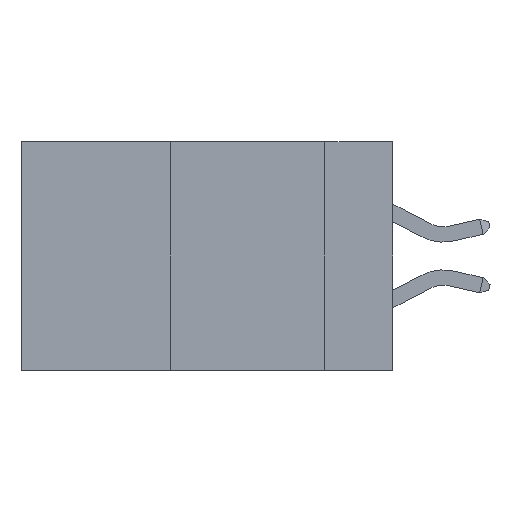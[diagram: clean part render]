
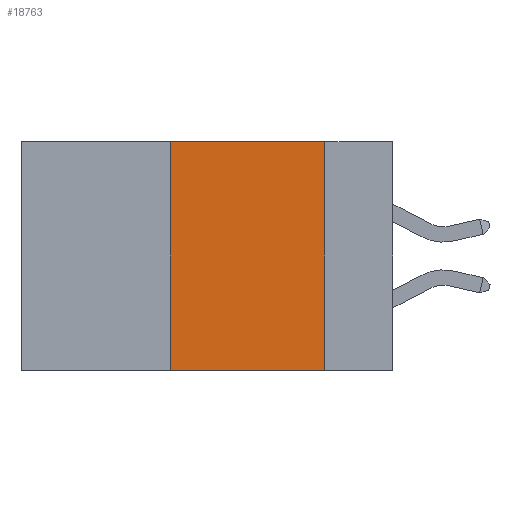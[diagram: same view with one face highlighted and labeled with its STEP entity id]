
A CAD part, left-side view. The second image highlights one B-rep face of the part: STEP entity #18763.
In plain terms, the highlighted planar face has unit normal (-1, 0, 0).
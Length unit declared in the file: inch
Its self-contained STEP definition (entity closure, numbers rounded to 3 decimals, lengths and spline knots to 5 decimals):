
#264 = VERTEX_POINT ( 'NONE', #22663 ) ;
#1376 = DIRECTION ( 'NONE',  ( 1., 0., 0. ) ) ;
#3195 = CARTESIAN_POINT ( 'NONE',  ( 0., 0.36, 0. ) ) ;
#3597 = CARTESIAN_POINT ( 'NONE',  ( 0., 0.6, -0.37 ) ) ;
#4513 = DIRECTION ( 'NONE',  ( 0., 0., -1. ) ) ;
#4616 = LINE ( 'NONE', #3597, #22181 ) ;
#5320 = VECTOR ( 'NONE', #4513, 39.37008 ) ;
#5803 = EDGE_CURVE ( 'NONE', #264, #16401, #4616, .T. ) ;
#6816 = AXIS2_PLACEMENT_3D ( 'NONE', #20392, #1376, #9915 ) ;
#7433 = CARTESIAN_POINT ( 'NONE',  ( 0., 0.11, 0. ) ) ;
#7488 = VECTOR ( 'NONE', #25372, 39.37008 ) ;
#7644 = VERTEX_POINT ( 'NONE', #3195 ) ;
#8243 = CARTESIAN_POINT ( 'NONE',  ( 0., 0.36, 0. ) ) ;
#8740 = VECTOR ( 'NONE', #18044, 39.37008 ) ;
#9915 = DIRECTION ( 'NONE',  ( 0., 0., -1. ) ) ;
#10943 = LINE ( 'NONE', #25445, #5320 ) ;
#11496 = VERTEX_POINT ( 'NONE', #7433 ) ;
#13374 = EDGE_LOOP ( 'NONE', ( #26297, #23035, #20560, #19013 ) ) ;
#13442 = CARTESIAN_POINT ( 'NONE',  ( 0., 0.11, -0.37 ) ) ;
#14347 = LINE ( 'NONE', #24248, #8740 ) ;
#15193 = EDGE_CURVE ( 'NONE', #11496, #16401, #10943, .T. ) ;
#16401 = VERTEX_POINT ( 'NONE', #13442 ) ;
#18044 = DIRECTION ( 'NONE',  ( 0., -1., 0. ) ) ;
#18763 = ADVANCED_FACE ( 'NONE', ( #23980 ), #22612, .F. ) ;
#19013 = ORIENTED_EDGE ( 'NONE', *, *, #5803, .T. ) ;
#19242 = EDGE_CURVE ( 'NONE', #7644, #11496, #14347, .T. ) ;
#20392 = CARTESIAN_POINT ( 'NONE',  ( 0., 0.6, 0. ) ) ;
#20560 = ORIENTED_EDGE ( 'NONE', *, *, #23405, .F. ) ;
#20727 = LINE ( 'NONE', #8243, #7488 ) ;
#22181 = VECTOR ( 'NONE', #23232, 39.37008 ) ;
#22612 = PLANE ( 'NONE',  #6816 ) ;
#22663 = CARTESIAN_POINT ( 'NONE',  ( 0., 0.36, -0.37 ) ) ;
#23035 = ORIENTED_EDGE ( 'NONE', *, *, #19242, .F. ) ;
#23232 = DIRECTION ( 'NONE',  ( 0., -1., 0. ) ) ;
#23405 = EDGE_CURVE ( 'NONE', #264, #7644, #20727, .T. ) ;
#23980 = FACE_OUTER_BOUND ( 'NONE', #13374, .T. ) ;
#24248 = CARTESIAN_POINT ( 'NONE',  ( 0., 0.6, 0. ) ) ;
#25372 = DIRECTION ( 'NONE',  ( 0., 0., 1. ) ) ;
#25445 = CARTESIAN_POINT ( 'NONE',  ( 0., 0.11, 0. ) ) ;
#26297 = ORIENTED_EDGE ( 'NONE', *, *, #15193, .F. ) ;
